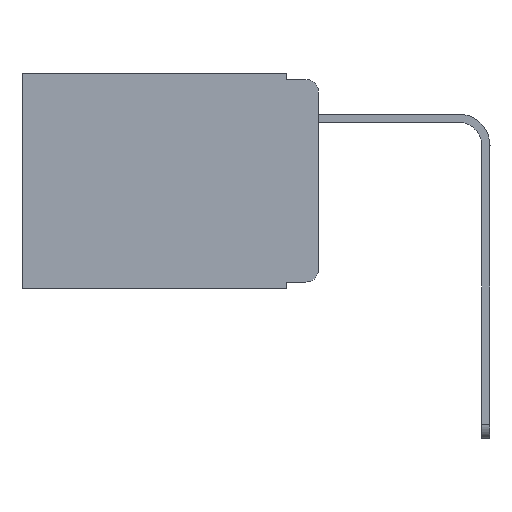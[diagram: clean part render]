
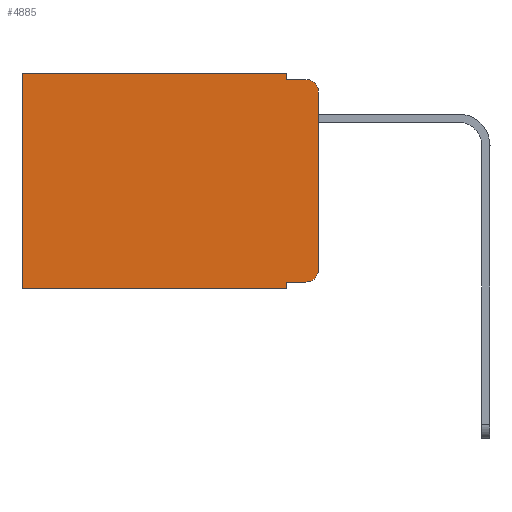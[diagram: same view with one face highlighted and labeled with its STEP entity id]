
A CAD part, left-side view. The second image highlights one B-rep face of the part: STEP entity #4885.
In plain terms, the highlighted planar face has unit normal (-1, 0, 0).
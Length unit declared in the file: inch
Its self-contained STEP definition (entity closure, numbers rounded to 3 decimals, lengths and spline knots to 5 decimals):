
#2 = CARTESIAN_POINT ( 'NONE',  ( 0.298, 0.051, -0.333 ) ) ;
#48 = ORIENTED_EDGE ( 'NONE', *, *, #5560, .F. ) ;
#64 = CARTESIAN_POINT ( 'NONE',  ( 0.298, 0.051, -0.01 ) ) ;
#102 = CIRCLE ( 'NONE', #6838, 0.02 ) ;
#295 = CARTESIAN_POINT ( 'NONE',  ( 0.298, 0.051, 0. ) ) ;
#332 = LINE ( 'NONE', #9666, #2462 ) ;
#409 = CARTESIAN_POINT ( 'NONE',  ( 0.298, 0.051, -0.343 ) ) ;
#425 = ORIENTED_EDGE ( 'NONE', *, *, #9897, .T. ) ;
#426 = CARTESIAN_POINT ( 'NONE',  ( 0.298, 0., 0. ) ) ;
#659 = DIRECTION ( 'NONE',  ( 1., 0., 0. ) ) ;
#716 = AXIS2_PLACEMENT_3D ( 'NONE', #5204, #1854, #909 ) ;
#909 = DIRECTION ( 'NONE',  ( 0., 0., -1. ) ) ;
#978 = ORIENTED_EDGE ( 'NONE', *, *, #10444, .T. ) ;
#1095 = EDGE_CURVE ( 'NONE', #9581, #8987, #102, .T. ) ;
#1498 = CARTESIAN_POINT ( 'NONE',  ( 0.298, 0., -0.03 ) ) ;
#1854 = DIRECTION ( 'NONE',  ( -1., 0., 0. ) ) ;
#2133 = ORIENTED_EDGE ( 'NONE', *, *, #8750, .T. ) ;
#2399 = EDGE_CURVE ( 'NONE', #9581, #6591, #8325, .T. ) ;
#2423 = CARTESIAN_POINT ( 'NONE',  ( 0.298, 0., 0. ) ) ;
#2462 = VECTOR ( 'NONE', #7944, 39.37008 ) ;
#2522 = DIRECTION ( 'NONE',  ( 0., 0., -1. ) ) ;
#3013 = ORIENTED_EDGE ( 'NONE', *, *, #1095, .T. ) ;
#3055 = VERTEX_POINT ( 'NONE', #10577 ) ;
#3104 = CARTESIAN_POINT ( 'NONE',  ( 0.298, 0., -0.313 ) ) ;
#3407 = LINE ( 'NONE', #4675, #9457 ) ;
#3881 = LINE ( 'NONE', #5049, #9805 ) ;
#3969 = VERTEX_POINT ( 'NONE', #2 ) ;
#4030 = LINE ( 'NONE', #426, #6806 ) ;
#4675 = CARTESIAN_POINT ( 'NONE',  ( 0.298, 0.473, 0. ) ) ;
#4681 = LINE ( 'NONE', #10544, #7723 ) ;
#4689 = ORIENTED_EDGE ( 'NONE', *, *, #2399, .F. ) ;
#4741 = VERTEX_POINT ( 'NONE', #5530 ) ;
#4885 = ADVANCED_FACE ( 'NONE', ( #10476 ), #10701, .F. ) ;
#4982 = ORIENTED_EDGE ( 'NONE', *, *, #7526, .F. ) ;
#5014 = CARTESIAN_POINT ( 'NONE',  ( 0.298, 0.02, -0.03 ) ) ;
#5049 = CARTESIAN_POINT ( 'NONE',  ( 0.298, 0.051, -0.01 ) ) ;
#5204 = CARTESIAN_POINT ( 'NONE',  ( 0.298, 0.02, -0.313 ) ) ;
#5371 = DIRECTION ( 'NONE',  ( 0., 0., -1. ) ) ;
#5530 = CARTESIAN_POINT ( 'NONE',  ( 0.298, 0.051, 0. ) ) ;
#5540 = ORIENTED_EDGE ( 'NONE', *, *, #6393, .F. ) ;
#5560 = EDGE_CURVE ( 'NONE', #3969, #10237, #10069, .T. ) ;
#5674 = DIRECTION ( 'NONE',  ( 0., 0., -1. ) ) ;
#5676 = VECTOR ( 'NONE', #6919, 39.37008 ) ;
#5856 = DIRECTION ( 'NONE',  ( -1., 0., 0. ) ) ;
#6075 = CARTESIAN_POINT ( 'NONE',  ( 0.298, 0., 0. ) ) ;
#6151 = VECTOR ( 'NONE', #5674, 39.37008 ) ;
#6307 = LINE ( 'NONE', #295, #9886 ) ;
#6343 = VERTEX_POINT ( 'NONE', #9964 ) ;
#6393 = EDGE_CURVE ( 'NONE', #10237, #7410, #332, .T. ) ;
#6465 = EDGE_CURVE ( 'NONE', #3969, #6343, #4681, .T. ) ;
#6591 = VERTEX_POINT ( 'NONE', #3104 ) ;
#6741 = DIRECTION ( 'NONE',  ( 0., -1., 0. ) ) ;
#6806 = VECTOR ( 'NONE', #7974, 39.37008 ) ;
#6838 = AXIS2_PLACEMENT_3D ( 'NONE', #5014, #5856, #2522 ) ;
#6919 = DIRECTION ( 'NONE',  ( 0., 0., -1. ) ) ;
#6933 = CARTESIAN_POINT ( 'NONE',  ( 0.298, 0.02, -0.01 ) ) ;
#7039 = CIRCLE ( 'NONE', #716, 0.02 ) ;
#7057 = ORIENTED_EDGE ( 'NONE', *, *, #6465, .T. ) ;
#7410 = VERTEX_POINT ( 'NONE', #7893 ) ;
#7526 = EDGE_CURVE ( 'NONE', #8045, #8987, #3881, .T. ) ;
#7723 = VECTOR ( 'NONE', #8033, 39.37008 ) ;
#7893 = CARTESIAN_POINT ( 'NONE',  ( 0.298, 0.473, -0.343 ) ) ;
#7944 = DIRECTION ( 'NONE',  ( 0., 1., 0. ) ) ;
#7974 = DIRECTION ( 'NONE',  ( 0., 1., 0. ) ) ;
#8033 = DIRECTION ( 'NONE',  ( 0., -1., 0. ) ) ;
#8045 = VERTEX_POINT ( 'NONE', #64 ) ;
#8101 = EDGE_CURVE ( 'NONE', #4741, #8045, #6307, .T. ) ;
#8283 = DIRECTION ( 'NONE',  ( 0., 0., -1. ) ) ;
#8325 = LINE ( 'NONE', #6075, #5676 ) ;
#8729 = DIRECTION ( 'NONE',  ( 0., 0., -1. ) ) ;
#8750 = EDGE_CURVE ( 'NONE', #3055, #7410, #3407, .T. ) ;
#8855 = EDGE_LOOP ( 'NONE', ( #4689, #3013, #4982, #10662, #425, #2133, #5540, #48, #7057, #978 ) ) ;
#8987 = VERTEX_POINT ( 'NONE', #6933 ) ;
#9000 = CARTESIAN_POINT ( 'NONE',  ( 0.298, 0.051, 0. ) ) ;
#9457 = VECTOR ( 'NONE', #5371, 39.37008 ) ;
#9581 = VERTEX_POINT ( 'NONE', #1498 ) ;
#9666 = CARTESIAN_POINT ( 'NONE',  ( 0.298, 0., -0.343 ) ) ;
#9805 = VECTOR ( 'NONE', #6741, 39.37008 ) ;
#9886 = VECTOR ( 'NONE', #8729, 39.37008 ) ;
#9897 = EDGE_CURVE ( 'NONE', #4741, #3055, #4030, .T. ) ;
#9964 = CARTESIAN_POINT ( 'NONE',  ( 0.298, 0.02, -0.333 ) ) ;
#10069 = LINE ( 'NONE', #9000, #6151 ) ;
#10237 = VERTEX_POINT ( 'NONE', #409 ) ;
#10444 = EDGE_CURVE ( 'NONE', #6343, #6591, #7039, .T. ) ;
#10476 = FACE_OUTER_BOUND ( 'NONE', #8855, .T. ) ;
#10544 = CARTESIAN_POINT ( 'NONE',  ( 0.298, 0.051, -0.333 ) ) ;
#10577 = CARTESIAN_POINT ( 'NONE',  ( 0.298, 0.473, 0. ) ) ;
#10662 = ORIENTED_EDGE ( 'NONE', *, *, #8101, .F. ) ;
#10697 = AXIS2_PLACEMENT_3D ( 'NONE', #2423, #659, #8283 ) ;
#10701 = PLANE ( 'NONE',  #10697 ) ;
